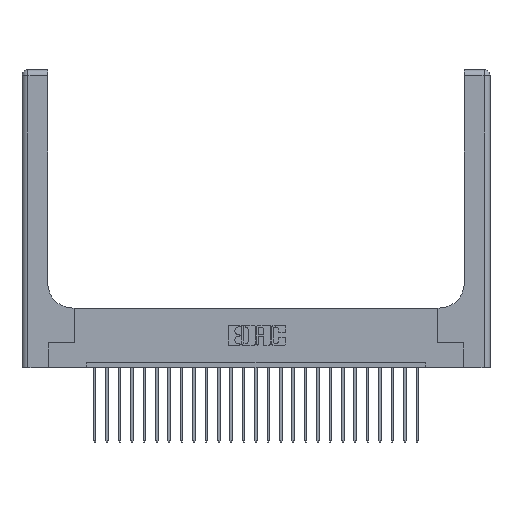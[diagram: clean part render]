
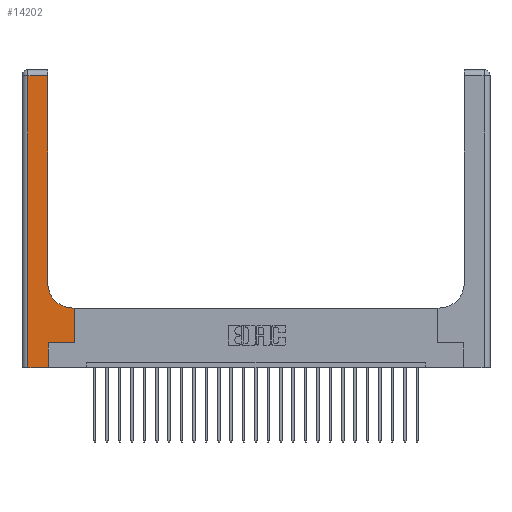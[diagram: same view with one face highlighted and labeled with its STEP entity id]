
A CAD part, top view. The second image highlights one B-rep face of the part: STEP entity #14202.
In plain terms, the highlighted planar face has unit normal (0, 0, 1).
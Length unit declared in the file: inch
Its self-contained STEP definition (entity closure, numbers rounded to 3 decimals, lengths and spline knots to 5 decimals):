
#345 = ORIENTED_EDGE ( 'NONE', *, *, #7581, .T. ) ;
#388 = CARTESIAN_POINT ( 'NONE',  ( 0.26, 3., 0.37 ) ) ;
#657 = CARTESIAN_POINT ( 'NONE',  ( 0.265, 0., 0.37 ) ) ;
#1160 = CARTESIAN_POINT ( 'NONE',  ( 0.528, 0.25, 0.37 ) ) ;
#1355 = LINE ( 'NONE', #657, #17551 ) ;
#2165 = ORIENTED_EDGE ( 'NONE', *, *, #15541, .T. ) ;
#2167 = CARTESIAN_POINT ( 'NONE',  ( 0.26, 0.6, 0.37 ) ) ;
#2284 = LINE ( 'NONE', #2167, #2569 ) ;
#2463 = EDGE_CURVE ( 'NONE', #11144, #22581, #23848, .T. ) ;
#2557 = VECTOR ( 'NONE', #21090, 39.37008 ) ;
#2569 = VECTOR ( 'NONE', #21286, 39.37008 ) ;
#2793 = VECTOR ( 'NONE', #14423, 39.37008 ) ;
#3535 = VECTOR ( 'NONE', #18176, 39.37008 ) ;
#3636 = VERTEX_POINT ( 'NONE', #10855 ) ;
#3697 = DIRECTION ( 'NONE',  ( 0., 0., -1. ) ) ;
#3789 = FACE_OUTER_BOUND ( 'NONE', #17123, .T. ) ;
#3913 = CARTESIAN_POINT ( 'NONE',  ( 0., 3., 0.37 ) ) ;
#3996 = CARTESIAN_POINT ( 'NONE',  ( 0.06, 0., 0.37 ) ) ;
#5171 = DIRECTION ( 'NONE',  ( 0., 1., 0. ) ) ;
#5174 = CIRCLE ( 'NONE', #14215, 0.25 ) ;
#5390 = LINE ( 'NONE', #7612, #9390 ) ;
#6817 = LINE ( 'NONE', #19905, #3535 ) ;
#6926 = VERTEX_POINT ( 'NONE', #11548 ) ;
#7250 = DIRECTION ( 'NONE',  ( 0., 0., -1. ) ) ;
#7283 = ORIENTED_EDGE ( 'NONE', *, *, #15878, .T. ) ;
#7360 = LINE ( 'NONE', #16857, #20054 ) ;
#7490 = DIRECTION ( 'NONE',  ( -1., 0., 0. ) ) ;
#7581 = EDGE_CURVE ( 'NONE', #19724, #16933, #13205, .T. ) ;
#7612 = CARTESIAN_POINT ( 'NONE',  ( 0., 2.94, 0.37 ) ) ;
#9026 = ORIENTED_EDGE ( 'NONE', *, *, #24259, .T. ) ;
#9390 = VECTOR ( 'NONE', #7490, 39.37008 ) ;
#9757 = DIRECTION ( 'NONE',  ( 0., 1., 0. ) ) ;
#10196 = LINE ( 'NONE', #13533, #2557 ) ;
#10855 = CARTESIAN_POINT ( 'NONE',  ( 0.51, 0.6, 0.37 ) ) ;
#10947 = DIRECTION ( 'NONE',  ( 0., 1., 0. ) ) ;
#11144 = VERTEX_POINT ( 'NONE', #15025 ) ;
#11318 = VERTEX_POINT ( 'NONE', #20979 ) ;
#11519 = EDGE_CURVE ( 'NONE', #22581, #22985, #7360, .T. ) ;
#11548 = CARTESIAN_POINT ( 'NONE',  ( 0.265, 0., 0.37 ) ) ;
#13205 = LINE ( 'NONE', #388, #14274 ) ;
#13533 = CARTESIAN_POINT ( 'NONE',  ( 0.06, 3., 0.37 ) ) ;
#13787 = ORIENTED_EDGE ( 'NONE', *, *, #16702, .T. ) ;
#13928 = CARTESIAN_POINT ( 'NONE',  ( 0.265, 0.25, 0.37 ) ) ;
#14202 = ADVANCED_FACE ( 'NONE', ( #3789 ), #24192, .F. ) ;
#14215 = AXIS2_PLACEMENT_3D ( 'NONE', #22602, #3697, #14798 ) ;
#14274 = VECTOR ( 'NONE', #9757, 39.37008 ) ;
#14335 = AXIS2_PLACEMENT_3D ( 'NONE', #3913, #7250, #22326 ) ;
#14423 = DIRECTION ( 'NONE',  ( 1., 0., 0. ) ) ;
#14798 = DIRECTION ( 'NONE',  ( 1., 0., 0. ) ) ;
#15025 = CARTESIAN_POINT ( 'NONE',  ( 0.265, 0.25, 0.37 ) ) ;
#15070 = ORIENTED_EDGE ( 'NONE', *, *, #2463, .T. ) ;
#15541 = EDGE_CURVE ( 'NONE', #11318, #18912, #10196, .T. ) ;
#15878 = EDGE_CURVE ( 'NONE', #22985, #3636, #2284, .T. ) ;
#16245 = CARTESIAN_POINT ( 'NONE',  ( 0.26, 0.85, 0.37 ) ) ;
#16702 = EDGE_CURVE ( 'NONE', #6926, #11144, #1355, .T. ) ;
#16857 = CARTESIAN_POINT ( 'NONE',  ( 0.528, 0.25, 0.37 ) ) ;
#16933 = VERTEX_POINT ( 'NONE', #22342 ) ;
#16996 = ORIENTED_EDGE ( 'NONE', *, *, #20493, .T. ) ;
#17123 = EDGE_LOOP ( 'NONE', ( #345, #16996, #2165, #19569, #13787, #15070, #18689, #7283, #9026 ) ) ;
#17415 = CARTESIAN_POINT ( 'NONE',  ( 0.528, 0.6, 0.37 ) ) ;
#17551 = VECTOR ( 'NONE', #5171, 39.37008 ) ;
#18176 = DIRECTION ( 'NONE',  ( 1., 0., 0. ) ) ;
#18689 = ORIENTED_EDGE ( 'NONE', *, *, #11519, .T. ) ;
#18912 = VERTEX_POINT ( 'NONE', #3996 ) ;
#19569 = ORIENTED_EDGE ( 'NONE', *, *, #22548, .T. ) ;
#19724 = VERTEX_POINT ( 'NONE', #16245 ) ;
#19905 = CARTESIAN_POINT ( 'NONE',  ( 0., 0., 0.37 ) ) ;
#20054 = VECTOR ( 'NONE', #10947, 39.37008 ) ;
#20493 = EDGE_CURVE ( 'NONE', #16933, #11318, #5390, .T. ) ;
#20979 = CARTESIAN_POINT ( 'NONE',  ( 0.06, 2.94, 0.37 ) ) ;
#21090 = DIRECTION ( 'NONE',  ( 0., -1., 0. ) ) ;
#21286 = DIRECTION ( 'NONE',  ( -1., 0., 0. ) ) ;
#22326 = DIRECTION ( 'NONE',  ( -1., 0., 0. ) ) ;
#22342 = CARTESIAN_POINT ( 'NONE',  ( 0.26, 2.94, 0.37 ) ) ;
#22548 = EDGE_CURVE ( 'NONE', #18912, #6926, #6817, .T. ) ;
#22581 = VERTEX_POINT ( 'NONE', #1160 ) ;
#22602 = CARTESIAN_POINT ( 'NONE',  ( 0.51, 0.85, 0.37 ) ) ;
#22985 = VERTEX_POINT ( 'NONE', #17415 ) ;
#23848 = LINE ( 'NONE', #13928, #2793 ) ;
#24192 = PLANE ( 'NONE',  #14335 ) ;
#24259 = EDGE_CURVE ( 'NONE', #3636, #19724, #5174, .T. ) ;
